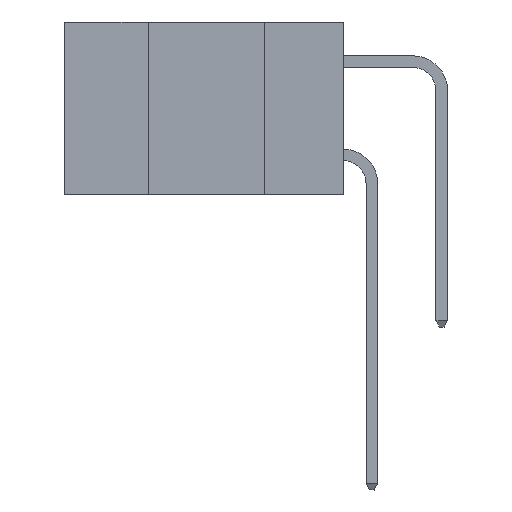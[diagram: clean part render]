
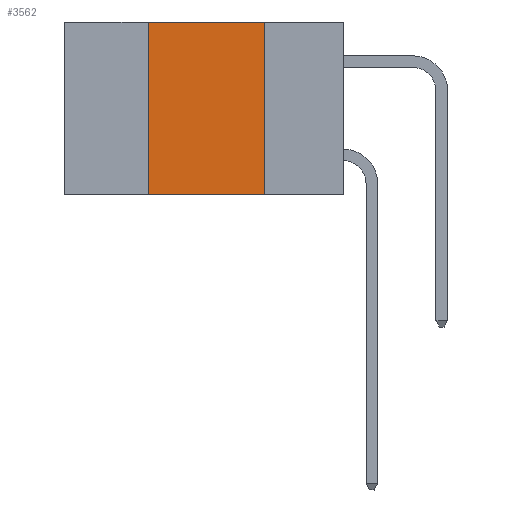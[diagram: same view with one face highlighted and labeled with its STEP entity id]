
A CAD part, left-side view. The second image highlights one B-rep face of the part: STEP entity #3562.
In plain terms, the highlighted planar face has unit normal (-1, 0, 0).
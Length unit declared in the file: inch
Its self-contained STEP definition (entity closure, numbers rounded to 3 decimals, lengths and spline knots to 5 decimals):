
#243 = CARTESIAN_POINT ( 'NONE',  ( 0., 0.42, 0. ) ) ;
#635 = EDGE_CURVE ( 'NONE', #2301, #10965, #3754, .T. ) ;
#1666 = EDGE_CURVE ( 'NONE', #2301, #3772, #12245, .T. ) ;
#1803 = DIRECTION ( 'NONE',  ( 1., 0., 0. ) ) ;
#2301 = VERTEX_POINT ( 'NONE', #17573 ) ;
#2585 = LINE ( 'NONE', #10446, #12799 ) ;
#2740 = CARTESIAN_POINT ( 'NONE',  ( 0., 0.42, -0.37 ) ) ;
#2849 = DIRECTION ( 'NONE',  ( 0., -1., 0. ) ) ;
#3562 = ADVANCED_FACE ( 'NONE', ( #11354 ), #9834, .F. ) ;
#3754 = LINE ( 'NONE', #2740, #12063 ) ;
#3772 = VERTEX_POINT ( 'NONE', #17356 ) ;
#3792 = ORIENTED_EDGE ( 'NONE', *, *, #11401, .F. ) ;
#4065 = LINE ( 'NONE', #6723, #8764 ) ;
#4076 = VERTEX_POINT ( 'NONE', #14101 ) ;
#4127 = CARTESIAN_POINT ( 'NONE',  ( 0., 0.6, -0.37 ) ) ;
#5529 = VECTOR ( 'NONE', #2849, 39.37008 ) ;
#5652 = DIRECTION ( 'NONE',  ( 0., 0., -1. ) ) ;
#6723 = CARTESIAN_POINT ( 'NONE',  ( 0., 0.17, -0.37 ) ) ;
#6759 = DIRECTION ( 'NONE',  ( 0., 0., 1. ) ) ;
#6792 = AXIS2_PLACEMENT_3D ( 'NONE', #8485, #1803, #15281 ) ;
#7777 = DIRECTION ( 'NONE',  ( 0., -1., 0. ) ) ;
#8485 = CARTESIAN_POINT ( 'NONE',  ( 0., 0.6, 0. ) ) ;
#8757 = ORIENTED_EDGE ( 'NONE', *, *, #14630, .F. ) ;
#8764 = VECTOR ( 'NONE', #5652, 39.37008 ) ;
#8951 = EDGE_LOOP ( 'NONE', ( #3792, #8757, #14057, #9378 ) ) ;
#9378 = ORIENTED_EDGE ( 'NONE', *, *, #1666, .T. ) ;
#9834 = PLANE ( 'NONE',  #6792 ) ;
#10446 = CARTESIAN_POINT ( 'NONE',  ( 0., 0.6, 0. ) ) ;
#10965 = VERTEX_POINT ( 'NONE', #243 ) ;
#11354 = FACE_OUTER_BOUND ( 'NONE', #8951, .T. ) ;
#11401 = EDGE_CURVE ( 'NONE', #4076, #3772, #4065, .T. ) ;
#12063 = VECTOR ( 'NONE', #6759, 39.37008 ) ;
#12245 = LINE ( 'NONE', #4127, #5529 ) ;
#12799 = VECTOR ( 'NONE', #7777, 39.37008 ) ;
#14057 = ORIENTED_EDGE ( 'NONE', *, *, #635, .F. ) ;
#14101 = CARTESIAN_POINT ( 'NONE',  ( 0., 0.17, 0. ) ) ;
#14630 = EDGE_CURVE ( 'NONE', #10965, #4076, #2585, .T. ) ;
#15281 = DIRECTION ( 'NONE',  ( 0., 0., -1. ) ) ;
#17356 = CARTESIAN_POINT ( 'NONE',  ( 0., 0.17, -0.37 ) ) ;
#17573 = CARTESIAN_POINT ( 'NONE',  ( 0., 0.42, -0.37 ) ) ;
